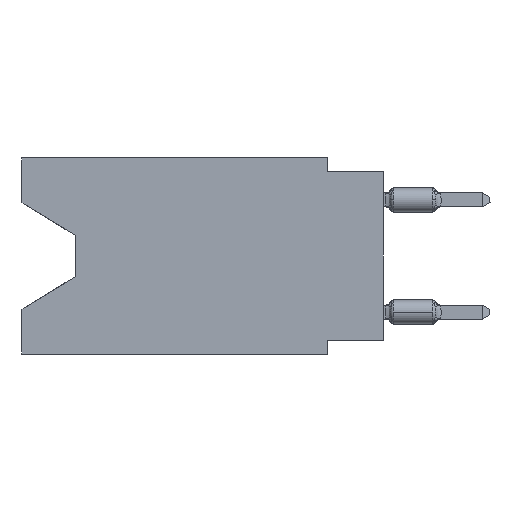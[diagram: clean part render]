
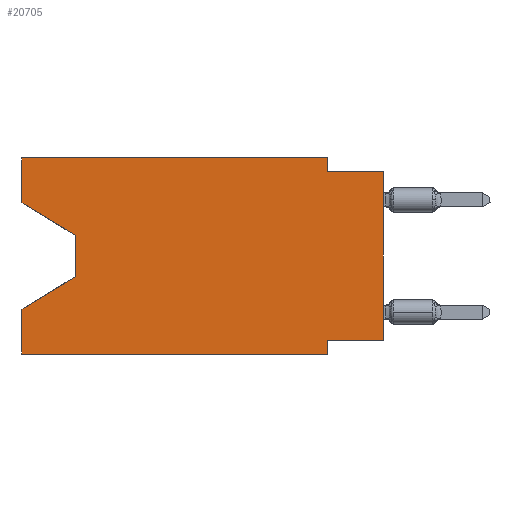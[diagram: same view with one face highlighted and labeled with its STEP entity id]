
A CAD part, left-side view. The second image highlights one B-rep face of the part: STEP entity #20705.
In plain terms, the highlighted planar face has unit normal (-1, 0, 0).
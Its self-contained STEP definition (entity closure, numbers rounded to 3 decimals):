
#124 = LINE ( 'NONE', #14451, #11397 ) ;
#855 = ORIENTED_EDGE ( 'NONE', *, *, #12833, .T. ) ;
#1504 = LINE ( 'NONE', #19532, #20681 ) ;
#1530 = DIRECTION ( 'NONE',  ( 0., 0., 1. ) ) ;
#1755 = LINE ( 'NONE', #8861, #9361 ) ;
#2662 = VECTOR ( 'NONE', #21970, 1000. ) ;
#2826 = ORIENTED_EDGE ( 'NONE', *, *, #21126, .F. ) ;
#2959 = CARTESIAN_POINT ( 'NONE',  ( 0., 2.54, -8.89 ) ) ;
#3250 = VERTEX_POINT ( 'NONE', #8213 ) ;
#3796 = DIRECTION ( 'NONE',  ( 0., 1., 0. ) ) ;
#4471 = LINE ( 'NONE', #6369, #19625 ) ;
#4685 = CARTESIAN_POINT ( 'NONE',  ( 0., 2.54, 0. ) ) ;
#4906 = EDGE_CURVE ( 'NONE', #20445, #13083, #7250, .T. ) ;
#5241 = CARTESIAN_POINT ( 'NONE',  ( 0., 16.383, 0. ) ) ;
#5285 = EDGE_CURVE ( 'NONE', #13083, #19832, #124, .T. ) ;
#5629 = LINE ( 'NONE', #16543, #19640 ) ;
#5911 = DIRECTION ( 'NONE',  ( 0., 0., 1. ) ) ;
#6292 = CARTESIAN_POINT ( 'NONE',  ( 0., 16.383, -8.89 ) ) ;
#6369 = CARTESIAN_POINT ( 'NONE',  ( 0., 0., -0.635 ) ) ;
#6475 = DIRECTION ( 'NONE',  ( 0., 0., 1. ) ) ;
#6678 = VERTEX_POINT ( 'NONE', #2959 ) ;
#7068 = DIRECTION ( 'NONE',  ( 0., 0., -1. ) ) ;
#7250 = LINE ( 'NONE', #20188, #2662 ) ;
#7334 = CARTESIAN_POINT ( 'NONE',  ( 0., 2.54, -0.635 ) ) ;
#7357 = CARTESIAN_POINT ( 'NONE',  ( 0., 0., -8.255 ) ) ;
#7491 = VECTOR ( 'NONE', #19476, 1000. ) ;
#7534 = CARTESIAN_POINT ( 'NONE',  ( 0., 13.97, -3.505 ) ) ;
#8191 = LINE ( 'NONE', #6292, #21543 ) ;
#8213 = CARTESIAN_POINT ( 'NONE',  ( 0., 16.383, 0. ) ) ;
#8424 = CARTESIAN_POINT ( 'NONE',  ( 0., 16.383, -2.038 ) ) ;
#8673 = LINE ( 'NONE', #19830, #7491 ) ;
#8698 = DIRECTION ( 'NONE',  ( 0., 0., -1. ) ) ;
#8861 = CARTESIAN_POINT ( 'NONE',  ( 0., 16.383, 0. ) ) ;
#8951 = CARTESIAN_POINT ( 'NONE',  ( 0., 0., -0.635 ) ) ;
#9012 = VECTOR ( 'NONE', #5911, 1000. ) ;
#9097 = AXIS2_PLACEMENT_3D ( 'NONE', #5241, #19852, #8698 ) ;
#9124 = DIRECTION ( 'NONE',  ( 0., 0.855, -0.519 ) ) ;
#9328 = EDGE_CURVE ( 'NONE', #10777, #13859, #22971, .T. ) ;
#9361 = VECTOR ( 'NONE', #1530, 1000. ) ;
#9635 = VECTOR ( 'NONE', #6475, 1000. ) ;
#9991 = ORIENTED_EDGE ( 'NONE', *, *, #4906, .T. ) ;
#10152 = CARTESIAN_POINT ( 'NONE',  ( 0., 0., 0. ) ) ;
#10281 = VERTEX_POINT ( 'NONE', #22048 ) ;
#10457 = ORIENTED_EDGE ( 'NONE', *, *, #9328, .T. ) ;
#10708 = EDGE_CURVE ( 'NONE', #20582, #3250, #10899, .T. ) ;
#10777 = VERTEX_POINT ( 'NONE', #13265 ) ;
#10899 = LINE ( 'NONE', #14918, #9012 ) ;
#11152 = LINE ( 'NONE', #7357, #11219 ) ;
#11219 = VECTOR ( 'NONE', #3796, 1000. ) ;
#11397 = VECTOR ( 'NONE', #9124, 1000. ) ;
#11525 = EDGE_CURVE ( 'NONE', #10281, #6678, #8191, .T. ) ;
#12404 = ORIENTED_EDGE ( 'NONE', *, *, #10708, .F. ) ;
#12545 = CARTESIAN_POINT ( 'NONE',  ( 0., 16.383, -6.852 ) ) ;
#12833 = EDGE_CURVE ( 'NONE', #20582, #20445, #17444, .T. ) ;
#13083 = VERTEX_POINT ( 'NONE', #14812 ) ;
#13265 = CARTESIAN_POINT ( 'NONE',  ( 0., 0., -8.255 ) ) ;
#13322 = EDGE_CURVE ( 'NONE', #10281, #19832, #1755, .T. ) ;
#13647 = DIRECTION ( 'NONE',  ( 0., -1., 0. ) ) ;
#13738 = ORIENTED_EDGE ( 'NONE', *, *, #21081, .F. ) ;
#13859 = VERTEX_POINT ( 'NONE', #8951 ) ;
#14451 = CARTESIAN_POINT ( 'NONE',  ( 0., 13.97, -5.385 ) ) ;
#14606 = FACE_OUTER_BOUND ( 'NONE', #22847, .T. ) ;
#14758 = ORIENTED_EDGE ( 'NONE', *, *, #13322, .F. ) ;
#14812 = CARTESIAN_POINT ( 'NONE',  ( 0., 13.97, -5.385 ) ) ;
#14918 = CARTESIAN_POINT ( 'NONE',  ( 0., 16.383, 0. ) ) ;
#15661 = DIRECTION ( 'NONE',  ( 0., -0.855, -0.519 ) ) ;
#16543 = CARTESIAN_POINT ( 'NONE',  ( 0., 2.54, -8.89 ) ) ;
#17444 = LINE ( 'NONE', #8424, #18819 ) ;
#17859 = DIRECTION ( 'NONE',  ( 0., -1., 0. ) ) ;
#18616 = ORIENTED_EDGE ( 'NONE', *, *, #19509, .F. ) ;
#18819 = VECTOR ( 'NONE', #15661, 1000. ) ;
#19022 = VERTEX_POINT ( 'NONE', #19996 ) ;
#19053 = EDGE_CURVE ( 'NONE', #3250, #20195, #1504, .T. ) ;
#19391 = CARTESIAN_POINT ( 'NONE',  ( 0., 16.383, -2.038 ) ) ;
#19476 = DIRECTION ( 'NONE',  ( 0., 0., -1. ) ) ;
#19509 = EDGE_CURVE ( 'NONE', #10777, #19022, #11152, .T. ) ;
#19532 = CARTESIAN_POINT ( 'NONE',  ( 0., 16.383, 0. ) ) ;
#19625 = VECTOR ( 'NONE', #22174, 1000. ) ;
#19640 = VECTOR ( 'NONE', #7068, 1000. ) ;
#19830 = CARTESIAN_POINT ( 'NONE',  ( 0., 2.54, 0. ) ) ;
#19832 = VERTEX_POINT ( 'NONE', #12545 ) ;
#19852 = DIRECTION ( 'NONE',  ( 1., 0., 0. ) ) ;
#19996 = CARTESIAN_POINT ( 'NONE',  ( 0., 2.54, -8.255 ) ) ;
#20188 = CARTESIAN_POINT ( 'NONE',  ( 0., 13.97, -3.505 ) ) ;
#20195 = VERTEX_POINT ( 'NONE', #4685 ) ;
#20445 = VERTEX_POINT ( 'NONE', #7534 ) ;
#20582 = VERTEX_POINT ( 'NONE', #19391 ) ;
#20681 = VECTOR ( 'NONE', #17859, 1000. ) ;
#20705 = ADVANCED_FACE ( 'NONE', ( #14606 ), #21865, .F. ) ;
#21081 = EDGE_CURVE ( 'NONE', #20195, #23086, #8673, .T. ) ;
#21126 = EDGE_CURVE ( 'NONE', #23086, #13859, #4471, .T. ) ;
#21277 = ORIENTED_EDGE ( 'NONE', *, *, #19053, .F. ) ;
#21406 = EDGE_CURVE ( 'NONE', #19022, #6678, #5629, .T. ) ;
#21458 = ORIENTED_EDGE ( 'NONE', *, *, #21406, .F. ) ;
#21543 = VECTOR ( 'NONE', #13647, 1000. ) ;
#21865 = PLANE ( 'NONE',  #9097 ) ;
#21970 = DIRECTION ( 'NONE',  ( 0., 0., -1. ) ) ;
#22048 = CARTESIAN_POINT ( 'NONE',  ( 0., 16.383, -8.89 ) ) ;
#22174 = DIRECTION ( 'NONE',  ( 0., -1., 0. ) ) ;
#22847 = EDGE_LOOP ( 'NONE', ( #855, #9991, #22984, #14758, #23376, #21458, #18616, #10457, #2826, #13738, #21277, #12404 ) ) ;
#22971 = LINE ( 'NONE', #10152, #9635 ) ;
#22984 = ORIENTED_EDGE ( 'NONE', *, *, #5285, .T. ) ;
#23086 = VERTEX_POINT ( 'NONE', #7334 ) ;
#23376 = ORIENTED_EDGE ( 'NONE', *, *, #11525, .T. ) ;
